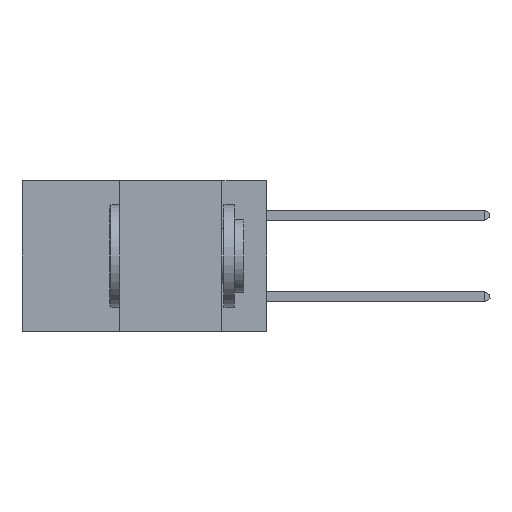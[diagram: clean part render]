
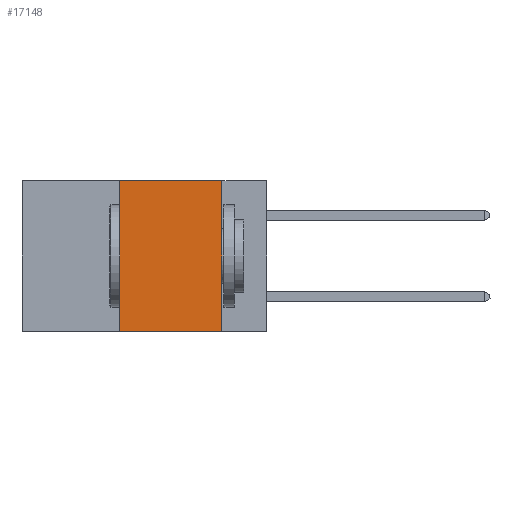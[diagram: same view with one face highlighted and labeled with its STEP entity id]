
A CAD part, left-side view. The second image highlights one B-rep face of the part: STEP entity #17148.
In plain terms, the highlighted planar face has unit normal (-1, 0, 0).
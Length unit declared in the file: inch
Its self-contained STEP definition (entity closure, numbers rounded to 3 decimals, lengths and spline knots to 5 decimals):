
#360 = EDGE_CURVE ( 'NONE', #2456, #3103, #18077, .T. ) ;
#526 = CARTESIAN_POINT ( 'NONE',  ( 0., 0.6, 0. ) ) ;
#1029 = DIRECTION ( 'NONE',  ( 0., -1., 0. ) ) ;
#1275 = CARTESIAN_POINT ( 'NONE',  ( 0., 0.11, 0. ) ) ;
#2166 = CARTESIAN_POINT ( 'NONE',  ( 0., 0.11, 0. ) ) ;
#2236 = CARTESIAN_POINT ( 'NONE',  ( 0., 0.6, -0.37 ) ) ;
#2310 = DIRECTION ( 'NONE',  ( 0., -1., 0. ) ) ;
#2322 = DIRECTION ( 'NONE',  ( 0., 0., 1. ) ) ;
#2456 = VERTEX_POINT ( 'NONE', #4411 ) ;
#3103 = VERTEX_POINT ( 'NONE', #12712 ) ;
#3149 = ORIENTED_EDGE ( 'NONE', *, *, #18419, .F. ) ;
#3813 = AXIS2_PLACEMENT_3D ( 'NONE', #5249, #17320, #7025 ) ;
#3897 = ORIENTED_EDGE ( 'NONE', *, *, #6805, .F. ) ;
#4411 = CARTESIAN_POINT ( 'NONE',  ( 0., 0.36, -0.37 ) ) ;
#4437 = CARTESIAN_POINT ( 'NONE',  ( 0., 0.36, 0. ) ) ;
#5249 = CARTESIAN_POINT ( 'NONE',  ( 0., 0.6, 0. ) ) ;
#6602 = ORIENTED_EDGE ( 'NONE', *, *, #360, .T. ) ;
#6805 = EDGE_CURVE ( 'NONE', #10822, #15927, #20039, .T. ) ;
#6929 = FACE_OUTER_BOUND ( 'NONE', #17806, .T. ) ;
#7025 = DIRECTION ( 'NONE',  ( 0., 0., -1. ) ) ;
#10822 = VERTEX_POINT ( 'NONE', #4437 ) ;
#11072 = VECTOR ( 'NONE', #2310, 39.37008 ) ;
#12043 = DIRECTION ( 'NONE',  ( 0., 0., -1. ) ) ;
#12712 = CARTESIAN_POINT ( 'NONE',  ( 0., 0.11, -0.37 ) ) ;
#12821 = EDGE_CURVE ( 'NONE', #2456, #10822, #19007, .T. ) ;
#13655 = VECTOR ( 'NONE', #1029, 39.37008 ) ;
#14762 = ORIENTED_EDGE ( 'NONE', *, *, #12821, .F. ) ;
#15149 = VECTOR ( 'NONE', #2322, 39.37008 ) ;
#15927 = VERTEX_POINT ( 'NONE', #2166 ) ;
#16416 = CARTESIAN_POINT ( 'NONE',  ( 0., 0.36, 0. ) ) ;
#17148 = ADVANCED_FACE ( 'NONE', ( #6929 ), #22348, .F. ) ;
#17320 = DIRECTION ( 'NONE',  ( 1., 0., 0. ) ) ;
#17806 = EDGE_LOOP ( 'NONE', ( #3149, #3897, #14762, #6602 ) ) ;
#18077 = LINE ( 'NONE', #2236, #13655 ) ;
#18419 = EDGE_CURVE ( 'NONE', #15927, #3103, #20814, .T. ) ;
#19007 = LINE ( 'NONE', #16416, #15149 ) ;
#20039 = LINE ( 'NONE', #526, #11072 ) ;
#20814 = LINE ( 'NONE', #1275, #21333 ) ;
#21333 = VECTOR ( 'NONE', #12043, 39.37008 ) ;
#22348 = PLANE ( 'NONE',  #3813 ) ;
